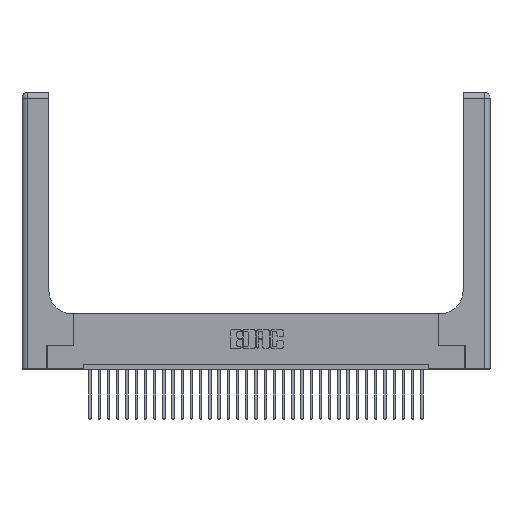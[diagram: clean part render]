
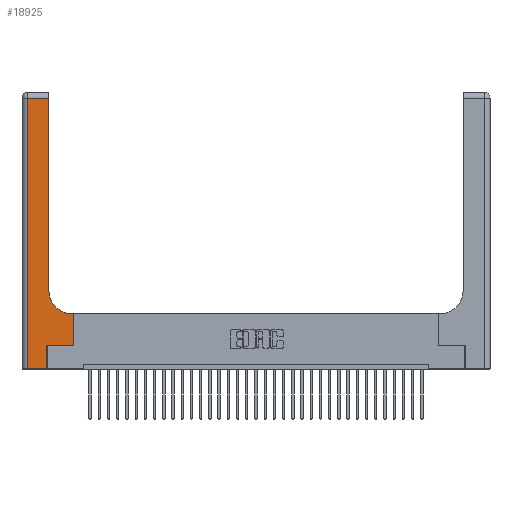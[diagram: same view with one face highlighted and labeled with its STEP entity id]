
A CAD part, top view. The second image highlights one B-rep face of the part: STEP entity #18925.
In plain terms, the highlighted planar face has unit normal (0, 0, 1).
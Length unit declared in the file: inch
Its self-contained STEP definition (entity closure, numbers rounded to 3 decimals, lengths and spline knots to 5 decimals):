
#1611 = LINE ( 'NONE', #17000, #25614 ) ;
#2352 = DIRECTION ( 'NONE',  ( 1., 0., 0. ) ) ;
#2481 = VERTEX_POINT ( 'NONE', #3471 ) ;
#2500 = LINE ( 'NONE', #3915, #32728 ) ;
#3127 = CARTESIAN_POINT ( 'NONE',  ( 0., 3., 0.37 ) ) ;
#3471 = CARTESIAN_POINT ( 'NONE',  ( 0.06, 0., 0.37 ) ) ;
#3619 = CARTESIAN_POINT ( 'NONE',  ( 0.5585, 0.25, 0.37 ) ) ;
#3915 = CARTESIAN_POINT ( 'NONE',  ( 0.06, 3., 0.37 ) ) ;
#3977 = VERTEX_POINT ( 'NONE', #22389 ) ;
#3985 = EDGE_CURVE ( 'NONE', #3977, #6654, #29921, .T. ) ;
#4214 = ORIENTED_EDGE ( 'NONE', *, *, #17273, .T. ) ;
#4283 = CARTESIAN_POINT ( 'NONE',  ( 0.269, 0., 0.37 ) ) ;
#5547 = CARTESIAN_POINT ( 'NONE',  ( 0.5585, 0.25, 0.37 ) ) ;
#5754 = VERTEX_POINT ( 'NONE', #3619 ) ;
#6654 = VERTEX_POINT ( 'NONE', #15072 ) ;
#6691 = VERTEX_POINT ( 'NONE', #15295 ) ;
#6906 = VERTEX_POINT ( 'NONE', #10809 ) ;
#9099 = ORIENTED_EDGE ( 'NONE', *, *, #19687, .T. ) ;
#9138 = VECTOR ( 'NONE', #17502, 39.37008 ) ;
#9504 = CARTESIAN_POINT ( 'NONE',  ( 0.2915, 0.6, 0.37 ) ) ;
#10185 = VERTEX_POINT ( 'NONE', #25579 ) ;
#10568 = CARTESIAN_POINT ( 'NONE',  ( 0., 2.94, 0.37 ) ) ;
#10733 = PLANE ( 'NONE',  #11132 ) ;
#10807 = DIRECTION ( 'NONE',  ( -1., 0., 0. ) ) ;
#10809 = CARTESIAN_POINT ( 'NONE',  ( 0.06, 2.94, 0.37 ) ) ;
#10895 = CARTESIAN_POINT ( 'NONE',  ( 0.5415, 0.85, 0.37 ) ) ;
#11132 = AXIS2_PLACEMENT_3D ( 'NONE', #3127, #23855, #29071 ) ;
#11428 = VERTEX_POINT ( 'NONE', #18730 ) ;
#12004 = ORIENTED_EDGE ( 'NONE', *, *, #28246, .T. ) ;
#12115 = DIRECTION ( 'NONE',  ( -1., 0., 0. ) ) ;
#12904 = ORIENTED_EDGE ( 'NONE', *, *, #28941, .T. ) ;
#15052 = CARTESIAN_POINT ( 'NONE',  ( 0.2915, 3., 0.37 ) ) ;
#15072 = CARTESIAN_POINT ( 'NONE',  ( 0.269, 0.25, 0.37 ) ) ;
#15295 = CARTESIAN_POINT ( 'NONE',  ( 0.2915, 2.94, 0.37 ) ) ;
#16129 = EDGE_CURVE ( 'NONE', #10185, #11428, #27687, .T. ) ;
#16361 = LINE ( 'NONE', #20383, #24556 ) ;
#16540 = EDGE_LOOP ( 'NONE', ( #9099, #12904, #12004, #23211, #32556, #25175, #26232, #24823, #4214 ) ) ;
#17000 = CARTESIAN_POINT ( 'NONE',  ( 0., 0., 0.37 ) ) ;
#17154 = VECTOR ( 'NONE', #25708, 39.37008 ) ;
#17273 = EDGE_CURVE ( 'NONE', #11428, #22615, #32977, .T. ) ;
#17349 = EDGE_CURVE ( 'NONE', #5754, #10185, #32301, .T. ) ;
#17502 = DIRECTION ( 'NONE',  ( 0., 1., 0. ) ) ;
#18730 = CARTESIAN_POINT ( 'NONE',  ( 0.5415, 0.6, 0.37 ) ) ;
#18925 = ADVANCED_FACE ( 'NONE', ( #31587 ), #10733, .F. ) ;
#19687 = EDGE_CURVE ( 'NONE', #22615, #6691, #19752, .T. ) ;
#19752 = LINE ( 'NONE', #15052, #28642 ) ;
#20032 = VECTOR ( 'NONE', #10807, 39.37008 ) ;
#20383 = CARTESIAN_POINT ( 'NONE',  ( 0.269, 0.25, 0.37 ) ) ;
#20537 = EDGE_CURVE ( 'NONE', #6654, #5754, #16361, .T. ) ;
#20755 = VECTOR ( 'NONE', #12115, 39.37008 ) ;
#22389 = CARTESIAN_POINT ( 'NONE',  ( 0.269, 0., 0.37 ) ) ;
#22615 = VERTEX_POINT ( 'NONE', #24212 ) ;
#23123 = DIRECTION ( 'NONE',  ( 1., 0., 0. ) ) ;
#23211 = ORIENTED_EDGE ( 'NONE', *, *, #30437, .T. ) ;
#23855 = DIRECTION ( 'NONE',  ( 0., 0., -1. ) ) ;
#23911 = DIRECTION ( 'NONE',  ( 0., 0., -1. ) ) ;
#24212 = CARTESIAN_POINT ( 'NONE',  ( 0.2915, 0.85, 0.37 ) ) ;
#24500 = LINE ( 'NONE', #10568, #20032 ) ;
#24556 = VECTOR ( 'NONE', #2352, 39.37008 ) ;
#24652 = DIRECTION ( 'NONE',  ( 0., -1., 0. ) ) ;
#24823 = ORIENTED_EDGE ( 'NONE', *, *, #16129, .T. ) ;
#25175 = ORIENTED_EDGE ( 'NONE', *, *, #20537, .T. ) ;
#25579 = CARTESIAN_POINT ( 'NONE',  ( 0.5585, 0.6, 0.37 ) ) ;
#25614 = VECTOR ( 'NONE', #27821, 39.37008 ) ;
#25708 = DIRECTION ( 'NONE',  ( 0., 1., 0. ) ) ;
#26232 = ORIENTED_EDGE ( 'NONE', *, *, #17349, .T. ) ;
#27687 = LINE ( 'NONE', #9504, #20755 ) ;
#27821 = DIRECTION ( 'NONE',  ( 1., 0., 0. ) ) ;
#28246 = EDGE_CURVE ( 'NONE', #6906, #2481, #2500, .T. ) ;
#28642 = VECTOR ( 'NONE', #33708, 39.37008 ) ;
#28941 = EDGE_CURVE ( 'NONE', #6691, #6906, #24500, .T. ) ;
#29071 = DIRECTION ( 'NONE',  ( -1., 0., 0. ) ) ;
#29463 = AXIS2_PLACEMENT_3D ( 'NONE', #10895, #23911, #23123 ) ;
#29921 = LINE ( 'NONE', #4283, #9138 ) ;
#30437 = EDGE_CURVE ( 'NONE', #2481, #3977, #1611, .T. ) ;
#31587 = FACE_OUTER_BOUND ( 'NONE', #16540, .T. ) ;
#32301 = LINE ( 'NONE', #5547, #17154 ) ;
#32556 = ORIENTED_EDGE ( 'NONE', *, *, #3985, .T. ) ;
#32728 = VECTOR ( 'NONE', #24652, 39.37008 ) ;
#32977 = CIRCLE ( 'NONE', #29463, 0.25 ) ;
#33708 = DIRECTION ( 'NONE',  ( 0., 1., 0. ) ) ;
